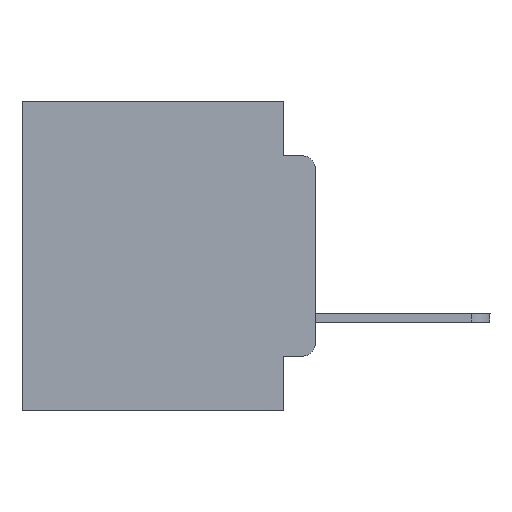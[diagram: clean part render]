
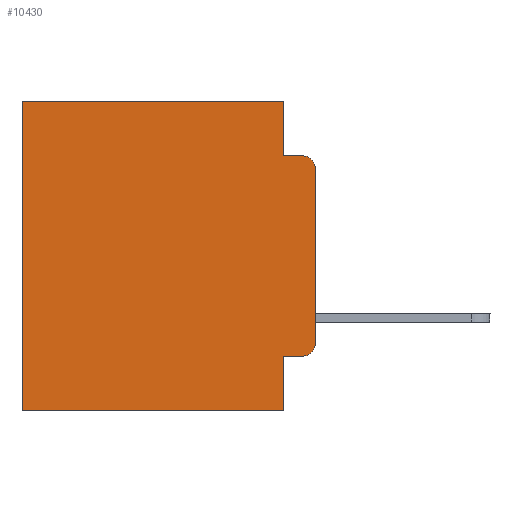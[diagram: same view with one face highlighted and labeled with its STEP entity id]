
A CAD part, left-side view. The second image highlights one B-rep face of the part: STEP entity #10430.
In plain terms, the highlighted planar face has unit normal (-1, 0, 0).
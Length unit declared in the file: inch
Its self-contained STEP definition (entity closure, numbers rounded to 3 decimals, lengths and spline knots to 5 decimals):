
#1350 = EDGE_CURVE ( 'NONE', #20107, #2964, #24822, .T. ) ;
#1488 = VERTEX_POINT ( 'NONE', #11194 ) ;
#1558 = ORIENTED_EDGE ( 'NONE', *, *, #3745, .F. ) ;
#1562 = EDGE_CURVE ( 'NONE', #20107, #9963, #17262, .T. ) ;
#1612 = DIRECTION ( 'NONE',  ( 0., 0., -1. ) ) ;
#1655 = DIRECTION ( 'NONE',  ( 0., -1., 0. ) ) ;
#1840 = CARTESIAN_POINT ( 'NONE',  ( 0.298, 0., 0. ) ) ;
#2657 = VECTOR ( 'NONE', #26171, 39.37008 ) ;
#2924 = ORIENTED_EDGE ( 'NONE', *, *, #24967, .T. ) ;
#2964 = VERTEX_POINT ( 'NONE', #8687 ) ;
#3176 = EDGE_CURVE ( 'NONE', #23023, #21128, #22146, .T. ) ;
#3186 = DIRECTION ( 'NONE',  ( 0., 1., 0. ) ) ;
#3745 = EDGE_CURVE ( 'NONE', #1488, #8421, #4933, .T. ) ;
#3799 = DIRECTION ( 'NONE',  ( -1., 0., 0. ) ) ;
#4666 = AXIS2_PLACEMENT_3D ( 'NONE', #11412, #5454, #1612 ) ;
#4889 = LINE ( 'NONE', #8716, #9014 ) ;
#4933 = LINE ( 'NONE', #23036, #11219 ) ;
#5197 = VECTOR ( 'NONE', #21802, 39.37008 ) ;
#5419 = FACE_OUTER_BOUND ( 'NONE', #12379, .T. ) ;
#5454 = DIRECTION ( 'NONE',  ( -1., 0., 0. ) ) ;
#5821 = ORIENTED_EDGE ( 'NONE', *, *, #14295, .T. ) ;
#6627 = CARTESIAN_POINT ( 'NONE',  ( 0.298, 0.051, -0.4115 ) ) ;
#6754 = CARTESIAN_POINT ( 'NONE',  ( 0.298, 0.02, -0.4115 ) ) ;
#7222 = VERTEX_POINT ( 'NONE', #22835 ) ;
#7480 = DIRECTION ( 'NONE',  ( 0., 0., -1. ) ) ;
#8091 = AXIS2_PLACEMENT_3D ( 'NONE', #1840, #23799, #9521 ) ;
#8421 = VERTEX_POINT ( 'NONE', #18644 ) ;
#8687 = CARTESIAN_POINT ( 'NONE',  ( 0.298, 0.051, -0.0885 ) ) ;
#8716 = CARTESIAN_POINT ( 'NONE',  ( 0.298, 0.051, 0. ) ) ;
#9014 = VECTOR ( 'NONE', #22724, 39.37008 ) ;
#9225 = CARTESIAN_POINT ( 'NONE',  ( 0.298, 0., 0. ) ) ;
#9308 = VERTEX_POINT ( 'NONE', #11025 ) ;
#9365 = EDGE_CURVE ( 'NONE', #21128, #20672, #13949, .T. ) ;
#9521 = DIRECTION ( 'NONE',  ( 0., 0., -1. ) ) ;
#9592 = DIRECTION ( 'NONE',  ( 0., -1., 0. ) ) ;
#9800 = ORIENTED_EDGE ( 'NONE', *, *, #3176, .T. ) ;
#9963 = VERTEX_POINT ( 'NONE', #17752 ) ;
#10430 = ADVANCED_FACE ( 'NONE', ( #5419 ), #19956, .F. ) ;
#10610 = ORIENTED_EDGE ( 'NONE', *, *, #15651, .F. ) ;
#11025 = CARTESIAN_POINT ( 'NONE',  ( 0.298, 0.02, -0.0885 ) ) ;
#11194 = CARTESIAN_POINT ( 'NONE',  ( 0.298, 0.051, -0.5 ) ) ;
#11219 = VECTOR ( 'NONE', #3186, 39.37008 ) ;
#11412 = CARTESIAN_POINT ( 'NONE',  ( 0.298, 0.02, -0.3915 ) ) ;
#12379 = EDGE_LOOP ( 'NONE', ( #10610, #5821, #23075, #20489, #23750, #2924, #1558, #23289, #9800, #15300 ) ) ;
#12472 = VECTOR ( 'NONE', #7480, 39.37008 ) ;
#13857 = CARTESIAN_POINT ( 'NONE',  ( 0.298, 0.02, -0.1085 ) ) ;
#13949 = CIRCLE ( 'NONE', #4666, 0.02 ) ;
#14295 = EDGE_CURVE ( 'NONE', #7222, #9308, #22427, .T. ) ;
#14542 = VECTOR ( 'NONE', #1655, 39.37008 ) ;
#14854 = CARTESIAN_POINT ( 'NONE',  ( 0.298, 0., -0.3915 ) ) ;
#14887 = CARTESIAN_POINT ( 'NONE',  ( 0.298, 0., 0. ) ) ;
#15300 = ORIENTED_EDGE ( 'NONE', *, *, #9365, .T. ) ;
#15651 = EDGE_CURVE ( 'NONE', #7222, #20672, #21263, .T. ) ;
#17262 = LINE ( 'NONE', #14887, #20400 ) ;
#17752 = CARTESIAN_POINT ( 'NONE',  ( 0.298, 0.473, 0. ) ) ;
#17977 = CARTESIAN_POINT ( 'NONE',  ( 0.298, 0.051, 0. ) ) ;
#18644 = CARTESIAN_POINT ( 'NONE',  ( 0.298, 0.473, -0.5 ) ) ;
#19697 = CARTESIAN_POINT ( 'NONE',  ( 0.298, 0.051, 0. ) ) ;
#19804 = LINE ( 'NONE', #25909, #2657 ) ;
#19909 = CARTESIAN_POINT ( 'NONE',  ( 0.298, 0.051, -0.4115 ) ) ;
#19956 = PLANE ( 'NONE',  #8091 ) ;
#20107 = VERTEX_POINT ( 'NONE', #19697 ) ;
#20400 = VECTOR ( 'NONE', #21107, 39.37008 ) ;
#20489 = ORIENTED_EDGE ( 'NONE', *, *, #1350, .F. ) ;
#20672 = VERTEX_POINT ( 'NONE', #14854 ) ;
#21107 = DIRECTION ( 'NONE',  ( 0., 1., 0. ) ) ;
#21128 = VERTEX_POINT ( 'NONE', #6754 ) ;
#21263 = LINE ( 'NONE', #9225, #12472 ) ;
#21802 = DIRECTION ( 'NONE',  ( 0., 0., -1. ) ) ;
#22146 = LINE ( 'NONE', #19909, #14542 ) ;
#22258 = EDGE_CURVE ( 'NONE', #2964, #9308, #23732, .T. ) ;
#22427 = CIRCLE ( 'NONE', #25170, 0.02 ) ;
#22724 = DIRECTION ( 'NONE',  ( 0., 0., -1. ) ) ;
#22835 = CARTESIAN_POINT ( 'NONE',  ( 0.298, 0., -0.1085 ) ) ;
#22977 = DIRECTION ( 'NONE',  ( 0., 0., -1. ) ) ;
#23023 = VERTEX_POINT ( 'NONE', #6627 ) ;
#23036 = CARTESIAN_POINT ( 'NONE',  ( 0.298, 0., -0.5 ) ) ;
#23075 = ORIENTED_EDGE ( 'NONE', *, *, #22258, .F. ) ;
#23289 = ORIENTED_EDGE ( 'NONE', *, *, #24689, .F. ) ;
#23470 = CARTESIAN_POINT ( 'NONE',  ( 0.298, 0.051, -0.0885 ) ) ;
#23732 = LINE ( 'NONE', #23470, #24979 ) ;
#23750 = ORIENTED_EDGE ( 'NONE', *, *, #1562, .T. ) ;
#23799 = DIRECTION ( 'NONE',  ( 1., 0., 0. ) ) ;
#24689 = EDGE_CURVE ( 'NONE', #23023, #1488, #4889, .T. ) ;
#24822 = LINE ( 'NONE', #17977, #5197 ) ;
#24967 = EDGE_CURVE ( 'NONE', #9963, #8421, #19804, .T. ) ;
#24979 = VECTOR ( 'NONE', #9592, 39.37008 ) ;
#25170 = AXIS2_PLACEMENT_3D ( 'NONE', #13857, #3799, #22977 ) ;
#25909 = CARTESIAN_POINT ( 'NONE',  ( 0.298, 0.473, 0. ) ) ;
#26171 = DIRECTION ( 'NONE',  ( 0., 0., -1. ) ) ;
